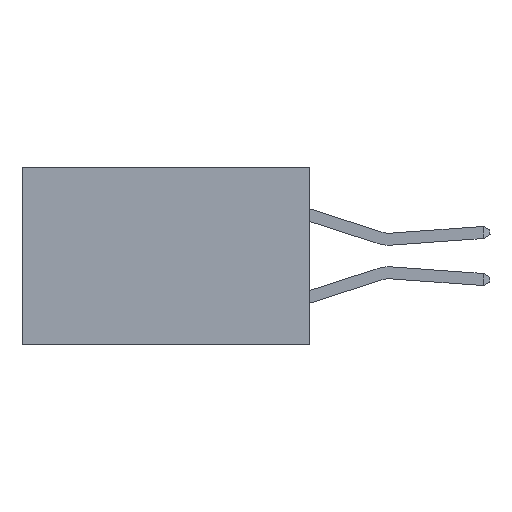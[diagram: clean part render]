
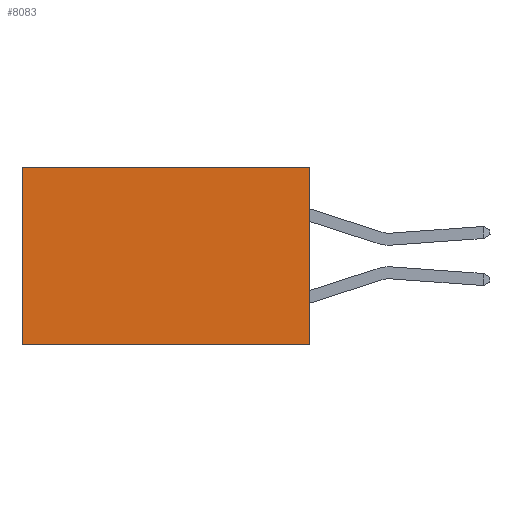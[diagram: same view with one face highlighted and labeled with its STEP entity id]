
A CAD part, left-side view. The second image highlights one B-rep face of the part: STEP entity #8083.
In plain terms, the highlighted planar face has unit normal (-1, 0, 0).
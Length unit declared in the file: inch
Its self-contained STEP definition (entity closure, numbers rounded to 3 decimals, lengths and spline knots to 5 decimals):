
#394 = CARTESIAN_POINT ( 'NONE',  ( 0.298, 0., 0. ) ) ;
#1776 = CARTESIAN_POINT ( 'NONE',  ( 0.298, 0., 0. ) ) ;
#1835 = CARTESIAN_POINT ( 'NONE',  ( 0.298, 0., -0.37 ) ) ;
#2397 = LINE ( 'NONE', #1776, #9678 ) ;
#6315 = ORIENTED_EDGE ( 'NONE', *, *, #12830, .T. ) ;
#7071 = CARTESIAN_POINT ( 'NONE',  ( 0.298, 0.6, 0. ) ) ;
#7563 = EDGE_CURVE ( 'NONE', #17614, #15336, #2397, .T. ) ;
#7695 = DIRECTION ( 'NONE',  ( 0., 0., -1. ) ) ;
#8083 = ADVANCED_FACE ( 'NONE', ( #12661 ), #17513, .F. ) ;
#8150 = DIRECTION ( 'NONE',  ( 0., 1., 0. ) ) ;
#8192 = CARTESIAN_POINT ( 'NONE',  ( 0.298, 0., -0.37 ) ) ;
#8242 = CARTESIAN_POINT ( 'NONE',  ( 0.298, 0.6, -0.37 ) ) ;
#8836 = CARTESIAN_POINT ( 'NONE',  ( 0.298, 0., 0. ) ) ;
#8838 = DIRECTION ( 'NONE',  ( 0., 0., -1. ) ) ;
#9023 = VERTEX_POINT ( 'NONE', #8242 ) ;
#9436 = LINE ( 'NONE', #8192, #16718 ) ;
#9678 = VECTOR ( 'NONE', #18695, 39.37008 ) ;
#9821 = ORIENTED_EDGE ( 'NONE', *, *, #18437, .F. ) ;
#10128 = CARTESIAN_POINT ( 'NONE',  ( 0.298, 0.6, 0. ) ) ;
#10154 = DIRECTION ( 'NONE',  ( 0., 0., -1. ) ) ;
#10335 = VECTOR ( 'NONE', #7695, 39.37008 ) ;
#11693 = CARTESIAN_POINT ( 'NONE',  ( 0.298, 0., 0. ) ) ;
#12458 = ORIENTED_EDGE ( 'NONE', *, *, #13068, .F. ) ;
#12661 = FACE_OUTER_BOUND ( 'NONE', #13546, .T. ) ;
#12830 = EDGE_CURVE ( 'NONE', #15336, #9023, #17825, .T. ) ;
#13068 = EDGE_CURVE ( 'NONE', #17224, #9023, #9436, .T. ) ;
#13252 = DIRECTION ( 'NONE',  ( 1., 0., 0. ) ) ;
#13463 = ORIENTED_EDGE ( 'NONE', *, *, #7563, .T. ) ;
#13546 = EDGE_LOOP ( 'NONE', ( #6315, #12458, #9821, #13463 ) ) ;
#13611 = VECTOR ( 'NONE', #10154, 39.37008 ) ;
#14721 = LINE ( 'NONE', #394, #10335 ) ;
#15336 = VERTEX_POINT ( 'NONE', #7071 ) ;
#16718 = VECTOR ( 'NONE', #8150, 39.37008 ) ;
#17224 = VERTEX_POINT ( 'NONE', #1835 ) ;
#17513 = PLANE ( 'NONE',  #18015 ) ;
#17614 = VERTEX_POINT ( 'NONE', #8836 ) ;
#17825 = LINE ( 'NONE', #10128, #13611 ) ;
#18015 = AXIS2_PLACEMENT_3D ( 'NONE', #11693, #13252, #8838 ) ;
#18437 = EDGE_CURVE ( 'NONE', #17614, #17224, #14721, .T. ) ;
#18695 = DIRECTION ( 'NONE',  ( 0., 1., 0. ) ) ;
